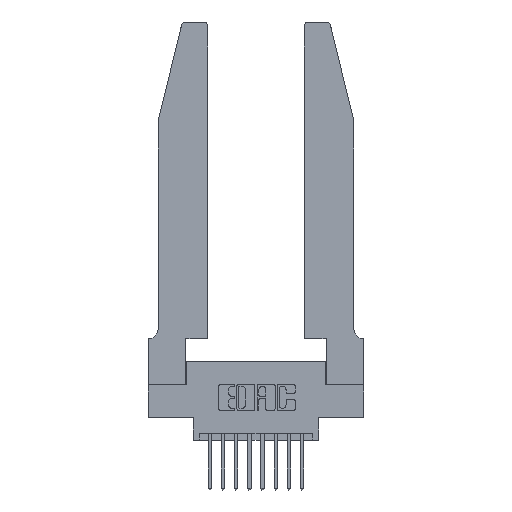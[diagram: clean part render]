
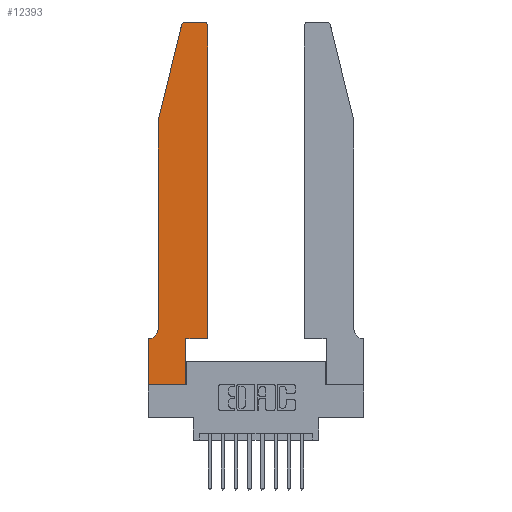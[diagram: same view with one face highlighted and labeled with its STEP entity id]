
A CAD part, top view. The second image highlights one B-rep face of the part: STEP entity #12393.
In plain terms, the highlighted planar face has unit normal (0, 0, 1).
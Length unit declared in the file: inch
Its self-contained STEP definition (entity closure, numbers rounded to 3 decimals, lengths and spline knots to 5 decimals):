
#27 = DIRECTION ( 'NONE',  ( 1., 0., 0. ) ) ;
#166 = EDGE_LOOP ( 'NONE', ( #632, #8562, #10480, #11726, #4998, #9198, #10650, #3535, #9817, #13537, #8886, #1885 ) ) ;
#469 = CARTESIAN_POINT ( 'NONE',  ( 0.4505, 0.35, 0.37 ) ) ;
#574 = EDGE_CURVE ( 'NONE', #7474, #8970, #12701, .T. ) ;
#632 = ORIENTED_EDGE ( 'NONE', *, *, #14403, .T. ) ;
#633 = DIRECTION ( 'NONE',  ( 1., 0., 0. ) ) ;
#799 = AXIS2_PLACEMENT_3D ( 'NONE', #4399, #12854, #5620 ) ;
#1343 = EDGE_CURVE ( 'NONE', #4791, #3655, #9259, .T. ) ;
#1427 = VECTOR ( 'NONE', #14812, 39.37008 ) ;
#1517 = VERTEX_POINT ( 'NONE', #6571 ) ;
#1792 = VERTEX_POINT ( 'NONE', #7280 ) ;
#1885 = ORIENTED_EDGE ( 'NONE', *, *, #574, .T. ) ;
#2087 = CIRCLE ( 'NONE', #13092, 0.03 ) ;
#2305 = CARTESIAN_POINT ( 'NONE',  ( 0., 0., 0.37 ) ) ;
#2330 = DIRECTION ( 'NONE',  ( 1., 0., 0. ) ) ;
#2362 = EDGE_CURVE ( 'NONE', #10206, #8194, #9981, .T. ) ;
#2590 = VECTOR ( 'NONE', #7489, 39.37008 ) ;
#2845 = VECTOR ( 'NONE', #2330, 39.37008 ) ;
#2933 = VERTEX_POINT ( 'NONE', #9884 ) ;
#3410 = DIRECTION ( 'NONE',  ( -1., 0., 0. ) ) ;
#3535 = ORIENTED_EDGE ( 'NONE', *, *, #2362, .T. ) ;
#3655 = VERTEX_POINT ( 'NONE', #3959 ) ;
#3699 = CARTESIAN_POINT ( 'NONE',  ( 0.2605, 2.75, 0.37 ) ) ;
#3839 = DIRECTION ( 'NONE',  ( 1., 0., 0. ) ) ;
#3841 = CARTESIAN_POINT ( 'NONE',  ( 0.4205, 2.72, 0.37 ) ) ;
#3897 = CARTESIAN_POINT ( 'NONE',  ( 0.0055, 0.42, 0.37 ) ) ;
#3959 = CARTESIAN_POINT ( 'NONE',  ( 0.4505, 0.35, 0.37 ) ) ;
#4155 = FACE_OUTER_BOUND ( 'NONE', #166, .T. ) ;
#4399 = CARTESIAN_POINT ( 'NONE',  ( 0., 0.35, 0.37 ) ) ;
#4695 = LINE ( 'NONE', #6394, #1427 ) ;
#4791 = VERTEX_POINT ( 'NONE', #9890 ) ;
#4998 = ORIENTED_EDGE ( 'NONE', *, *, #11604, .T. ) ;
#5099 = LINE ( 'NONE', #14645, #8328 ) ;
#5100 = DIRECTION ( 'NONE',  ( -1., 0., 0. ) ) ;
#5250 = VERTEX_POINT ( 'NONE', #8505 ) ;
#5620 = DIRECTION ( 'NONE',  ( 1., 0., 0. ) ) ;
#5785 = VECTOR ( 'NONE', #14580, 39.37008 ) ;
#5828 = VECTOR ( 'NONE', #10760, 39.37008 ) ;
#5902 = CARTESIAN_POINT ( 'NONE',  ( 0., 0.35, 0.37 ) ) ;
#6174 = CARTESIAN_POINT ( 'NONE',  ( 0.0755, 2., 0.37 ) ) ;
#6210 = EDGE_CURVE ( 'NONE', #1792, #9962, #13286, .T. ) ;
#6394 = CARTESIAN_POINT ( 'NONE',  ( 0.0755, 2., 0.37 ) ) ;
#6571 = CARTESIAN_POINT ( 'NONE',  ( 0.0755, 2., 0.37 ) ) ;
#6813 = VECTOR ( 'NONE', #633, 39.37008 ) ;
#6873 = EDGE_CURVE ( 'NONE', #5250, #2933, #2087, .T. ) ;
#6903 = VECTOR ( 'NONE', #12145, 39.37008 ) ;
#7280 = CARTESIAN_POINT ( 'NONE',  ( 0.0055, 0.35, 0.37 ) ) ;
#7442 = DIRECTION ( 'NONE',  ( 0., 0., 1. ) ) ;
#7447 = DIRECTION ( 'NONE',  ( 0., 1., 0. ) ) ;
#7474 = VERTEX_POINT ( 'NONE', #13465 ) ;
#7489 = DIRECTION ( 'NONE',  ( -0.239, -0.971, 0. ) ) ;
#8194 = VERTEX_POINT ( 'NONE', #10010 ) ;
#8328 = VECTOR ( 'NONE', #7447, 39.37008 ) ;
#8505 = CARTESIAN_POINT ( 'NONE',  ( 0.284, 2.75, 0.37 ) ) ;
#8562 = ORIENTED_EDGE ( 'NONE', *, *, #6873, .T. ) ;
#8654 = LINE ( 'NONE', #6174, #2590 ) ;
#8886 = ORIENTED_EDGE ( 'NONE', *, *, #10807, .T. ) ;
#8970 = VERTEX_POINT ( 'NONE', #10939 ) ;
#8979 = EDGE_CURVE ( 'NONE', #8194, #4791, #10085, .T. ) ;
#9198 = ORIENTED_EDGE ( 'NONE', *, *, #6210, .T. ) ;
#9259 = LINE ( 'NONE', #469, #2845 ) ;
#9480 = CARTESIAN_POINT ( 'NONE',  ( 0.0755, 0.35, 0.37 ) ) ;
#9551 = CARTESIAN_POINT ( 'NONE',  ( 0., 0., 0.37 ) ) ;
#9730 = CARTESIAN_POINT ( 'NONE',  ( 0.2865, 0.35, 0.37 ) ) ;
#9817 = ORIENTED_EDGE ( 'NONE', *, *, #8979, .T. ) ;
#9884 = CARTESIAN_POINT ( 'NONE',  ( 0.25487, 2.72718, 0.37 ) ) ;
#9890 = CARTESIAN_POINT ( 'NONE',  ( 0.2865, 0.35, 0.37 ) ) ;
#9962 = VERTEX_POINT ( 'NONE', #5902 ) ;
#9981 = LINE ( 'NONE', #2305, #6813 ) ;
#10010 = CARTESIAN_POINT ( 'NONE',  ( 0.2865, 0., 0.37 ) ) ;
#10085 = LINE ( 'NONE', #9730, #6903 ) ;
#10087 = VECTOR ( 'NONE', #3410, 39.37008 ) ;
#10206 = VERTEX_POINT ( 'NONE', #13511 ) ;
#10480 = ORIENTED_EDGE ( 'NONE', *, *, #13532, .T. ) ;
#10571 = CIRCLE ( 'NONE', #15054, 0.07 ) ;
#10650 = ORIENTED_EDGE ( 'NONE', *, *, #12987, .T. ) ;
#10760 = DIRECTION ( 'NONE',  ( 0., -1., 0. ) ) ;
#10807 = EDGE_CURVE ( 'NONE', #3655, #7474, #5099, .T. ) ;
#10939 = CARTESIAN_POINT ( 'NONE',  ( 0.4205, 2.75, 0.37 ) ) ;
#11604 = EDGE_CURVE ( 'NONE', #14493, #1792, #10571, .T. ) ;
#11726 = ORIENTED_EDGE ( 'NONE', *, *, #15154, .T. ) ;
#12145 = DIRECTION ( 'NONE',  ( 0., 1., 0. ) ) ;
#12333 = DIRECTION ( 'NONE',  ( 0., 0., -1. ) ) ;
#12393 = ADVANCED_FACE ( 'NONE', ( #4155 ), #15102, .T. ) ;
#12701 = CIRCLE ( 'NONE', #13914, 0.03 ) ;
#12854 = DIRECTION ( 'NONE',  ( 0., 0., 1. ) ) ;
#12987 = EDGE_CURVE ( 'NONE', #9962, #10206, #12998, .T. ) ;
#12998 = LINE ( 'NONE', #9551, #5828 ) ;
#13092 = AXIS2_PLACEMENT_3D ( 'NONE', #14640, #7442, #27 ) ;
#13286 = LINE ( 'NONE', #9480, #10087 ) ;
#13465 = CARTESIAN_POINT ( 'NONE',  ( 0.4505, 2.72, 0.37 ) ) ;
#13476 = CARTESIAN_POINT ( 'NONE',  ( 0.0755, 0.42, 0.37 ) ) ;
#13511 = CARTESIAN_POINT ( 'NONE',  ( 0., 0., 0.37 ) ) ;
#13532 = EDGE_CURVE ( 'NONE', #2933, #1517, #8654, .T. ) ;
#13537 = ORIENTED_EDGE ( 'NONE', *, *, #1343, .T. ) ;
#13914 = AXIS2_PLACEMENT_3D ( 'NONE', #3841, #15301, #3839 ) ;
#14403 = EDGE_CURVE ( 'NONE', #8970, #5250, #15387, .T. ) ;
#14493 = VERTEX_POINT ( 'NONE', #13476 ) ;
#14580 = DIRECTION ( 'NONE',  ( -1., 0., 0. ) ) ;
#14640 = CARTESIAN_POINT ( 'NONE',  ( 0.284, 2.72, 0.37 ) ) ;
#14645 = CARTESIAN_POINT ( 'NONE',  ( 0.4505, 0.35, 0.37 ) ) ;
#14812 = DIRECTION ( 'NONE',  ( 0., -1., 0. ) ) ;
#15054 = AXIS2_PLACEMENT_3D ( 'NONE', #3897, #12333, #5100 ) ;
#15102 = PLANE ( 'NONE',  #799 ) ;
#15154 = EDGE_CURVE ( 'NONE', #1517, #14493, #4695, .T. ) ;
#15301 = DIRECTION ( 'NONE',  ( 0., 0., 1. ) ) ;
#15387 = LINE ( 'NONE', #3699, #5785 ) ;
